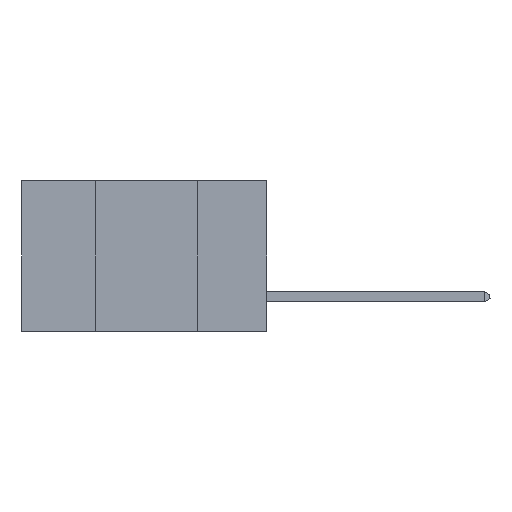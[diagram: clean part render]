
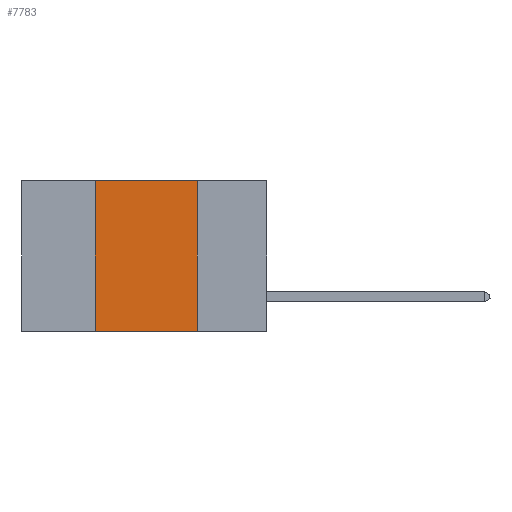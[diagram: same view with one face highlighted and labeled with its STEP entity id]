
A CAD part, left-side view. The second image highlights one B-rep face of the part: STEP entity #7783.
In plain terms, the highlighted planar face has unit normal (-1, 0, 0).
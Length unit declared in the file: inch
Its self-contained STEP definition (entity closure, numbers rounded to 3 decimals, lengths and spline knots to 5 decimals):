
#82 = DIRECTION ( 'NONE',  ( 0., -1., 0. ) ) ;
#194 = CARTESIAN_POINT ( 'NONE',  ( 0., 0.17, -0.37 ) ) ;
#674 = LINE ( 'NONE', #4153, #9586 ) ;
#716 = ORIENTED_EDGE ( 'NONE', *, *, #8303, .F. ) ;
#1527 = ORIENTED_EDGE ( 'NONE', *, *, #15942, .T. ) ;
#1811 = VECTOR ( 'NONE', #3302, 39.37008 ) ;
#2077 = CARTESIAN_POINT ( 'NONE',  ( 0., 0.17, 0. ) ) ;
#3004 = VERTEX_POINT ( 'NONE', #6131 ) ;
#3302 = DIRECTION ( 'NONE',  ( 0., 0., 1. ) ) ;
#4036 = LINE ( 'NONE', #9182, #1811 ) ;
#4153 = CARTESIAN_POINT ( 'NONE',  ( 0., 0.17, 0. ) ) ;
#4652 = VECTOR ( 'NONE', #82, 39.37008 ) ;
#4766 = VERTEX_POINT ( 'NONE', #6411 ) ;
#5681 = ORIENTED_EDGE ( 'NONE', *, *, #9084, .F. ) ;
#6113 = AXIS2_PLACEMENT_3D ( 'NONE', #9060, #12742, #8900 ) ;
#6131 = CARTESIAN_POINT ( 'NONE',  ( 0., 0.42, -0.37 ) ) ;
#6411 = CARTESIAN_POINT ( 'NONE',  ( 0., 0.42, 0. ) ) ;
#6582 = VERTEX_POINT ( 'NONE', #194 ) ;
#7081 = VERTEX_POINT ( 'NONE', #2077 ) ;
#7768 = PLANE ( 'NONE',  #6113 ) ;
#7783 = ADVANCED_FACE ( 'NONE', ( #15049 ), #7768, .F. ) ;
#7990 = LINE ( 'NONE', #11470, #14274 ) ;
#8303 = EDGE_CURVE ( 'NONE', #3004, #4766, #4036, .T. ) ;
#8900 = DIRECTION ( 'NONE',  ( 0., 0., -1. ) ) ;
#9060 = CARTESIAN_POINT ( 'NONE',  ( 0., 0.6, 0. ) ) ;
#9084 = EDGE_CURVE ( 'NONE', #4766, #7081, #12535, .T. ) ;
#9182 = CARTESIAN_POINT ( 'NONE',  ( 0., 0.42, 0. ) ) ;
#9586 = VECTOR ( 'NONE', #14192, 39.37008 ) ;
#10154 = EDGE_CURVE ( 'NONE', #7081, #6582, #674, .T. ) ;
#10254 = ORIENTED_EDGE ( 'NONE', *, *, #10154, .F. ) ;
#11470 = CARTESIAN_POINT ( 'NONE',  ( 0., 0.6, -0.37 ) ) ;
#11579 = DIRECTION ( 'NONE',  ( 0., -1., 0. ) ) ;
#12535 = LINE ( 'NONE', #12879, #4652 ) ;
#12742 = DIRECTION ( 'NONE',  ( 1., 0., 0. ) ) ;
#12879 = CARTESIAN_POINT ( 'NONE',  ( 0., 0.6, 0. ) ) ;
#13421 = EDGE_LOOP ( 'NONE', ( #10254, #5681, #716, #1527 ) ) ;
#14192 = DIRECTION ( 'NONE',  ( 0., 0., -1. ) ) ;
#14274 = VECTOR ( 'NONE', #11579, 39.37008 ) ;
#15049 = FACE_OUTER_BOUND ( 'NONE', #13421, .T. ) ;
#15942 = EDGE_CURVE ( 'NONE', #3004, #6582, #7990, .T. ) ;
